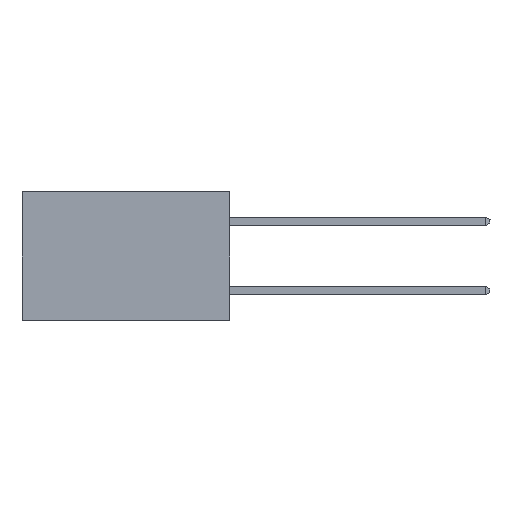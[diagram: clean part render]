
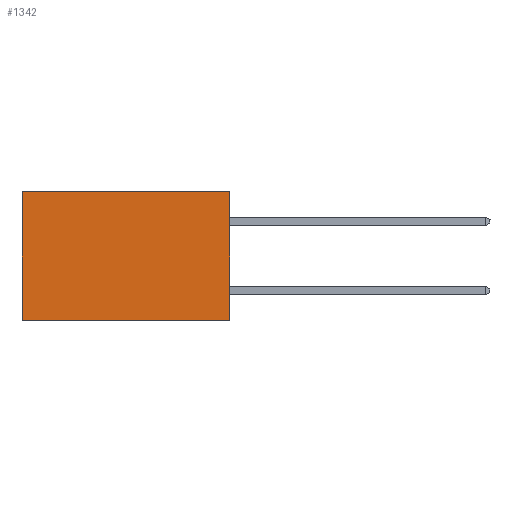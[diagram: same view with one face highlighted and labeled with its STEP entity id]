
A CAD part, left-side view. The second image highlights one B-rep face of the part: STEP entity #1342.
In plain terms, the highlighted planar face has unit normal (-1, 0, 0).
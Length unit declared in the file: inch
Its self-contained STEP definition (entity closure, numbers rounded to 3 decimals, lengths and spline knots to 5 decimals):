
#706 = CARTESIAN_POINT ( 'NONE',  ( 0.2615, 0., 0. ) ) ;
#744 = FACE_OUTER_BOUND ( 'NONE', #5286, .T. ) ;
#830 = LINE ( 'NONE', #7076, #4656 ) ;
#1342 = ADVANCED_FACE ( 'NONE', ( #744 ), #8263, .F. ) ;
#1490 = LINE ( 'NONE', #7602, #7970 ) ;
#1546 = CARTESIAN_POINT ( 'NONE',  ( 0.2615, 0., 0. ) ) ;
#1767 = EDGE_CURVE ( 'NONE', #3134, #7436, #4119, .T. ) ;
#2113 = DIRECTION ( 'NONE',  ( 0., 0., -1. ) ) ;
#2151 = ORIENTED_EDGE ( 'NONE', *, *, #4653, .T. ) ;
#2190 = AXIS2_PLACEMENT_3D ( 'NONE', #6936, #5479, #2113 ) ;
#2463 = CARTESIAN_POINT ( 'NONE',  ( 0.2615, 0.6, -0.37 ) ) ;
#2693 = DIRECTION ( 'NONE',  ( 0., 1., 0. ) ) ;
#2723 = DIRECTION ( 'NONE',  ( 0., 1., 0. ) ) ;
#3060 = VERTEX_POINT ( 'NONE', #1546 ) ;
#3134 = VERTEX_POINT ( 'NONE', #7615 ) ;
#3354 = EDGE_CURVE ( 'NONE', #3060, #5653, #8048, .T. ) ;
#3432 = VECTOR ( 'NONE', #2693, 39.37008 ) ;
#3588 = DIRECTION ( 'NONE',  ( 0., 0., -1. ) ) ;
#3992 = ORIENTED_EDGE ( 'NONE', *, *, #1767, .F. ) ;
#4119 = LINE ( 'NONE', #8073, #7020 ) ;
#4653 = EDGE_CURVE ( 'NONE', #5653, #7436, #830, .T. ) ;
#4656 = VECTOR ( 'NONE', #8409, 39.37008 ) ;
#5259 = ORIENTED_EDGE ( 'NONE', *, *, #8518, .F. ) ;
#5286 = EDGE_LOOP ( 'NONE', ( #2151, #3992, #5259, #8538 ) ) ;
#5479 = DIRECTION ( 'NONE',  ( 1., 0., 0. ) ) ;
#5653 = VERTEX_POINT ( 'NONE', #6177 ) ;
#6177 = CARTESIAN_POINT ( 'NONE',  ( 0.2615, 0.6, 0. ) ) ;
#6936 = CARTESIAN_POINT ( 'NONE',  ( 0.2615, 0., -0.37 ) ) ;
#7020 = VECTOR ( 'NONE', #2723, 39.37008 ) ;
#7076 = CARTESIAN_POINT ( 'NONE',  ( 0.2615, 0.6, -0.37 ) ) ;
#7436 = VERTEX_POINT ( 'NONE', #2463 ) ;
#7602 = CARTESIAN_POINT ( 'NONE',  ( 0.2615, 0., -0.37 ) ) ;
#7615 = CARTESIAN_POINT ( 'NONE',  ( 0.2615, 0., -0.37 ) ) ;
#7970 = VECTOR ( 'NONE', #3588, 39.37008 ) ;
#8048 = LINE ( 'NONE', #706, #3432 ) ;
#8073 = CARTESIAN_POINT ( 'NONE',  ( 0.2615, 0., -0.37 ) ) ;
#8263 = PLANE ( 'NONE',  #2190 ) ;
#8409 = DIRECTION ( 'NONE',  ( 0., 0., -1. ) ) ;
#8518 = EDGE_CURVE ( 'NONE', #3060, #3134, #1490, .T. ) ;
#8538 = ORIENTED_EDGE ( 'NONE', *, *, #3354, .T. ) ;
